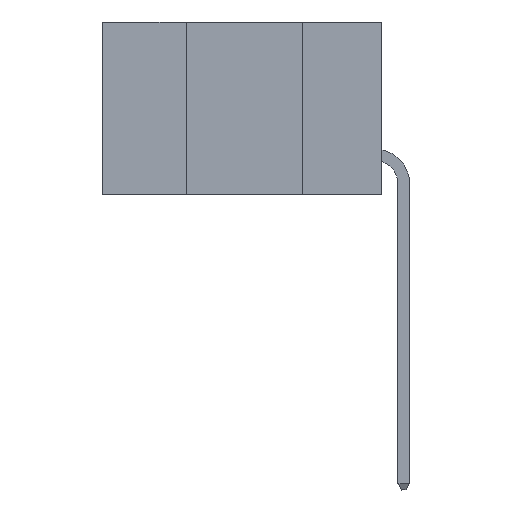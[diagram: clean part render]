
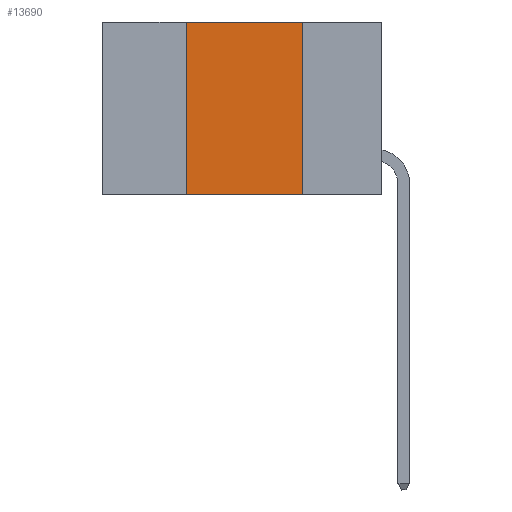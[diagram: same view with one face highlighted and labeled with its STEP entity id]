
A CAD part, left-side view. The second image highlights one B-rep face of the part: STEP entity #13690.
In plain terms, the highlighted planar face has unit normal (-1, 0, 0).
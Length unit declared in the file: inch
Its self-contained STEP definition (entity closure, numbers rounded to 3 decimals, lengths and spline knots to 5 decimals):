
#370 = VECTOR ( 'NONE', #17627, 39.37008 ) ;
#666 = CARTESIAN_POINT ( 'NONE',  ( 0., 0.6, 0. ) ) ;
#1146 = VECTOR ( 'NONE', #15821, 39.37008 ) ;
#1525 = VERTEX_POINT ( 'NONE', #11635 ) ;
#3542 = DIRECTION ( 'NONE',  ( 0., -1., 0. ) ) ;
#3631 = FACE_OUTER_BOUND ( 'NONE', #21535, .T. ) ;
#4708 = LINE ( 'NONE', #13712, #18854 ) ;
#5272 = ORIENTED_EDGE ( 'NONE', *, *, #21009, .F. ) ;
#6887 = VECTOR ( 'NONE', #3542, 39.37008 ) ;
#7039 = CARTESIAN_POINT ( 'NONE',  ( 0., 0.17, 0. ) ) ;
#9359 = DIRECTION ( 'NONE',  ( 1., 0., 0. ) ) ;
#9498 = CARTESIAN_POINT ( 'NONE',  ( 0., 0.42, -0.37 ) ) ;
#10752 = VERTEX_POINT ( 'NONE', #7039 ) ;
#11635 = CARTESIAN_POINT ( 'NONE',  ( 0., 0.42, 0. ) ) ;
#13690 = ADVANCED_FACE ( 'NONE', ( #3631 ), #16932, .F. ) ;
#13712 = CARTESIAN_POINT ( 'NONE',  ( 0., 0.42, 0. ) ) ;
#13861 = ORIENTED_EDGE ( 'NONE', *, *, #14827, .F. ) ;
#13868 = DIRECTION ( 'NONE',  ( 0., 0., 1. ) ) ;
#14025 = VERTEX_POINT ( 'NONE', #9498 ) ;
#14027 = CARTESIAN_POINT ( 'NONE',  ( 0., 0.17, -0.37 ) ) ;
#14214 = VERTEX_POINT ( 'NONE', #14027 ) ;
#14827 = EDGE_CURVE ( 'NONE', #14025, #1525, #4708, .T. ) ;
#15050 = CARTESIAN_POINT ( 'NONE',  ( 0., 0.6, -0.37 ) ) ;
#15517 = CARTESIAN_POINT ( 'NONE',  ( 0., 0.17, 0. ) ) ;
#15575 = EDGE_CURVE ( 'NONE', #10752, #14214, #17378, .T. ) ;
#15821 = DIRECTION ( 'NONE',  ( 0., 0., -1. ) ) ;
#16249 = ORIENTED_EDGE ( 'NONE', *, *, #15575, .F. ) ;
#16798 = ORIENTED_EDGE ( 'NONE', *, *, #20579, .T. ) ;
#16932 = PLANE ( 'NONE',  #20117 ) ;
#17282 = DIRECTION ( 'NONE',  ( 0., 0., -1. ) ) ;
#17378 = LINE ( 'NONE', #15517, #1146 ) ;
#17495 = LINE ( 'NONE', #15050, #6887 ) ;
#17627 = DIRECTION ( 'NONE',  ( 0., -1., 0. ) ) ;
#18528 = CARTESIAN_POINT ( 'NONE',  ( 0., 0.6, 0. ) ) ;
#18854 = VECTOR ( 'NONE', #13868, 39.37008 ) ;
#20117 = AXIS2_PLACEMENT_3D ( 'NONE', #18528, #9359, #17282 ) ;
#20579 = EDGE_CURVE ( 'NONE', #14025, #14214, #17495, .T. ) ;
#21009 = EDGE_CURVE ( 'NONE', #1525, #10752, #22768, .T. ) ;
#21535 = EDGE_LOOP ( 'NONE', ( #16249, #5272, #13861, #16798 ) ) ;
#22768 = LINE ( 'NONE', #666, #370 ) ;
